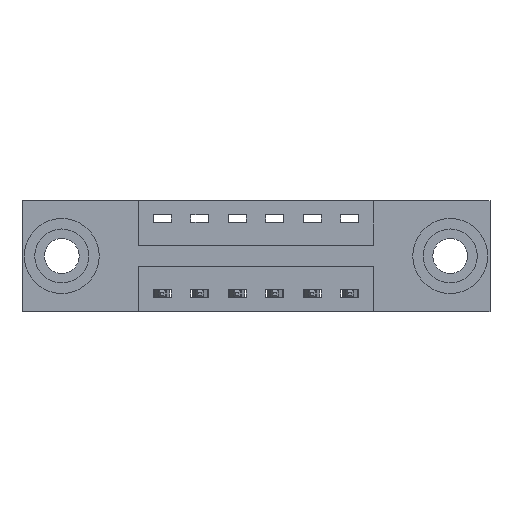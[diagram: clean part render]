
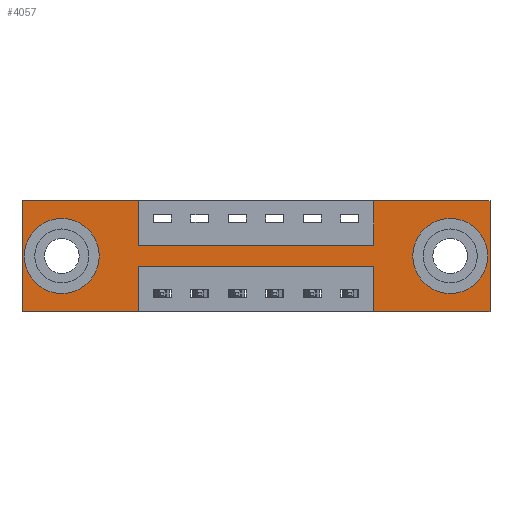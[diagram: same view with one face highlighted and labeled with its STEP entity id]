
A CAD part, front view. The second image highlights one B-rep face of the part: STEP entity #4057.
In plain terms, the highlighted planar face has unit normal (0, -1, 0).
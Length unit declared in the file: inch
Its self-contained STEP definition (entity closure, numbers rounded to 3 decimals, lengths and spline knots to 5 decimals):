
#3 = LINE ( 'NONE', #8240, #7728 ) ;
#8 = EDGE_CURVE ( 'NONE', #4295, #1855, #4288, .T. ) ;
#44 = FACE_OUTER_BOUND ( 'NONE', #9190, .T. ) ;
#78 = CARTESIAN_POINT ( 'NONE',  ( 1.4275, 0., -0.185 ) ) ;
#266 = EDGE_CURVE ( 'NONE', #8594, #5827, #3, .T. ) ;
#280 = LINE ( 'NONE', #2254, #2252 ) ;
#347 = AXIS2_PLACEMENT_3D ( 'NONE', #8436, #8417, #8403 ) ;
#463 = DIRECTION ( 'NONE',  ( 1., 0., 0. ) ) ;
#467 = LINE ( 'NONE', #4411, #4174 ) ;
#488 = LINE ( 'NONE', #4860, #4196 ) ;
#527 = VECTOR ( 'NONE', #7187, 39.37008 ) ;
#554 = CARTESIAN_POINT ( 'NONE',  ( 1.1725, 0., -0.37 ) ) ;
#571 = VERTEX_POINT ( 'NONE', #1957 ) ;
#653 = LINE ( 'NONE', #4208, #8131 ) ;
#664 = VERTEX_POINT ( 'NONE', #9116 ) ;
#706 = EDGE_CURVE ( 'NONE', #1855, #4295, #7501, .T. ) ;
#802 = CARTESIAN_POINT ( 'NONE',  ( 1.1725, 0., 0. ) ) ;
#817 = DIRECTION ( 'NONE',  ( 0., 0., -1. ) ) ;
#831 = ORIENTED_EDGE ( 'NONE', *, *, #8219, .F. ) ;
#1064 = ORIENTED_EDGE ( 'NONE', *, *, #6655, .F. ) ;
#1213 = EDGE_CURVE ( 'NONE', #1971, #5287, #467, .T. ) ;
#1297 = CARTESIAN_POINT ( 'NONE',  ( 0.3875, 0., -0.37 ) ) ;
#1302 = ORIENTED_EDGE ( 'NONE', *, *, #6002, .F. ) ;
#1307 = EDGE_LOOP ( 'NONE', ( #4530, #8278 ) ) ;
#1536 = ORIENTED_EDGE ( 'NONE', *, *, #266, .F. ) ;
#1554 = DIRECTION ( 'NONE',  ( 0., 0., 1. ) ) ;
#1693 = CARTESIAN_POINT ( 'NONE',  ( 1.4275, 0., -0.263 ) ) ;
#1702 = LINE ( 'NONE', #1297, #9037 ) ;
#1736 = AXIS2_PLACEMENT_3D ( 'NONE', #7558, #1827, #6892 ) ;
#1797 = VECTOR ( 'NONE', #4024, 39.37008 ) ;
#1799 = CARTESIAN_POINT ( 'NONE',  ( 0., 0., 0. ) ) ;
#1827 = DIRECTION ( 'NONE',  ( 0., -1., 0. ) ) ;
#1855 = VERTEX_POINT ( 'NONE', #7482 ) ;
#1957 = CARTESIAN_POINT ( 'NONE',  ( 1.1725, 0., -0.15 ) ) ;
#1971 = VERTEX_POINT ( 'NONE', #6198 ) ;
#2047 = LINE ( 'NONE', #802, #2281 ) ;
#2185 = CARTESIAN_POINT ( 'NONE',  ( 0.3875, 0., -0.22 ) ) ;
#2252 = VECTOR ( 'NONE', #2951, 39.37008 ) ;
#2254 = CARTESIAN_POINT ( 'NONE',  ( 0.3875, 0., -0.22 ) ) ;
#2281 = VECTOR ( 'NONE', #1554, 39.37008 ) ;
#2592 = ORIENTED_EDGE ( 'NONE', *, *, #7320, .T. ) ;
#2689 = EDGE_CURVE ( 'NONE', #5827, #7892, #6380, .T. ) ;
#2800 = DIRECTION ( 'NONE',  ( 0., 1., 0. ) ) ;
#2801 = ORIENTED_EDGE ( 'NONE', *, *, #5075, .F. ) ;
#2951 = DIRECTION ( 'NONE',  ( -1., 0., 0. ) ) ;
#3031 = CARTESIAN_POINT ( 'NONE',  ( 0., 0., -0.37 ) ) ;
#3075 = DIRECTION ( 'NONE',  ( 0., 0., -1. ) ) ;
#3173 = VECTOR ( 'NONE', #6745, 39.37008 ) ;
#3273 = ORIENTED_EDGE ( 'NONE', *, *, #3929, .F. ) ;
#3624 = VERTEX_POINT ( 'NONE', #1693 ) ;
#3750 = LINE ( 'NONE', #6861, #1797 ) ;
#3781 = DIRECTION ( 'NONE',  ( -1., 0., 0. ) ) ;
#3860 = AXIS2_PLACEMENT_3D ( 'NONE', #8392, #7022, #7272 ) ;
#3880 = CARTESIAN_POINT ( 'NONE',  ( 0.3875, 0., 0. ) ) ;
#3929 = EDGE_CURVE ( 'NONE', #7003, #8350, #8394, .T. ) ;
#3957 = CARTESIAN_POINT ( 'NONE',  ( 0., 0., -0.37 ) ) ;
#3998 = CARTESIAN_POINT ( 'NONE',  ( 1.56, 0., 0. ) ) ;
#4024 = DIRECTION ( 'NONE',  ( 0., 0., 1. ) ) ;
#4028 = EDGE_CURVE ( 'NONE', #9014, #664, #3750, .T. ) ;
#4051 = LINE ( 'NONE', #3031, #7604 ) ;
#4057 = ADVANCED_FACE ( 'NONE', ( #5455, #7319, #44 ), #5464, .T. ) ;
#4174 = VECTOR ( 'NONE', #4366, 39.37008 ) ;
#4196 = VECTOR ( 'NONE', #463, 39.37008 ) ;
#4208 = CARTESIAN_POINT ( 'NONE',  ( 0., 0., 0. ) ) ;
#4254 = EDGE_CURVE ( 'NONE', #5437, #3624, #7007, .T. ) ;
#4288 = CIRCLE ( 'NONE', #3860, 0.078 ) ;
#4295 = VERTEX_POINT ( 'NONE', #9176 ) ;
#4304 = ORIENTED_EDGE ( 'NONE', *, *, #4254, .T. ) ;
#4366 = DIRECTION ( 'NONE',  ( 1., 0., 0. ) ) ;
#4411 = CARTESIAN_POINT ( 'NONE',  ( 0., 0., 0. ) ) ;
#4530 = ORIENTED_EDGE ( 'NONE', *, *, #706, .T. ) ;
#4860 = CARTESIAN_POINT ( 'NONE',  ( 0.3875, 0., -0.15 ) ) ;
#4975 = ORIENTED_EDGE ( 'NONE', *, *, #5700, .F. ) ;
#4984 = CARTESIAN_POINT ( 'NONE',  ( 1.56, 0., -0.37 ) ) ;
#4988 = AXIS2_PLACEMENT_3D ( 'NONE', #78, #5219, #817 ) ;
#5005 = VERTEX_POINT ( 'NONE', #2185 ) ;
#5075 = EDGE_CURVE ( 'NONE', #664, #5005, #280, .T. ) ;
#5198 = VECTOR ( 'NONE', #3075, 39.37008 ) ;
#5200 = ORIENTED_EDGE ( 'NONE', *, *, #6098, .F. ) ;
#5219 = DIRECTION ( 'NONE',  ( 0., 1., 0. ) ) ;
#5287 = VERTEX_POINT ( 'NONE', #3998 ) ;
#5437 = VERTEX_POINT ( 'NONE', #7661 ) ;
#5455 = FACE_BOUND ( 'NONE', #6465, .T. ) ;
#5464 = PLANE ( 'NONE',  #1736 ) ;
#5700 = EDGE_CURVE ( 'NONE', #5287, #8225, #6663, .T. ) ;
#5827 = VERTEX_POINT ( 'NONE', #3957 ) ;
#6002 = EDGE_CURVE ( 'NONE', #8350, #571, #488, .T. ) ;
#6028 = CARTESIAN_POINT ( 'NONE',  ( 0.3875, 0., -0.37 ) ) ;
#6098 = EDGE_CURVE ( 'NONE', #7892, #7003, #653, .T. ) ;
#6198 = CARTESIAN_POINT ( 'NONE',  ( 1.1725, 0., 0. ) ) ;
#6380 = LINE ( 'NONE', #7225, #527 ) ;
#6465 = EDGE_LOOP ( 'NONE', ( #4304, #2592 ) ) ;
#6655 = EDGE_CURVE ( 'NONE', #8225, #9014, #4051, .T. ) ;
#6663 = LINE ( 'NONE', #7371, #5198 ) ;
#6664 = ORIENTED_EDGE ( 'NONE', *, *, #4028, .F. ) ;
#6745 = DIRECTION ( 'NONE',  ( 0., 0., -1. ) ) ;
#6861 = CARTESIAN_POINT ( 'NONE',  ( 1.1725, 0., -0.37 ) ) ;
#6884 = ORIENTED_EDGE ( 'NONE', *, *, #1213, .F. ) ;
#6892 = DIRECTION ( 'NONE',  ( 0., 0., -1. ) ) ;
#7003 = VERTEX_POINT ( 'NONE', #9045 ) ;
#7007 = CIRCLE ( 'NONE', #7992, 0.078 ) ;
#7022 = DIRECTION ( 'NONE',  ( 0., 1., 0. ) ) ;
#7128 = CARTESIAN_POINT ( 'NONE',  ( 1.4275, 0., -0.185 ) ) ;
#7137 = DIRECTION ( 'NONE',  ( 0., 0., -1. ) ) ;
#7187 = DIRECTION ( 'NONE',  ( 0., 0., 1. ) ) ;
#7190 = CARTESIAN_POINT ( 'NONE',  ( 0.3875, 0., -0.15 ) ) ;
#7225 = CARTESIAN_POINT ( 'NONE',  ( 0., 0., 0. ) ) ;
#7272 = DIRECTION ( 'NONE',  ( 0., 0., 1. ) ) ;
#7319 = FACE_BOUND ( 'NONE', #1307, .T. ) ;
#7320 = EDGE_CURVE ( 'NONE', #3624, #5437, #7478, .T. ) ;
#7371 = CARTESIAN_POINT ( 'NONE',  ( 1.56, 0., 0. ) ) ;
#7478 = CIRCLE ( 'NONE', #4988, 0.078 ) ;
#7482 = CARTESIAN_POINT ( 'NONE',  ( 0.1325, 0., -0.107 ) ) ;
#7501 = CIRCLE ( 'NONE', #347, 0.078 ) ;
#7558 = CARTESIAN_POINT ( 'NONE',  ( 0., 0., -0.37 ) ) ;
#7604 = VECTOR ( 'NONE', #3781, 39.37008 ) ;
#7661 = CARTESIAN_POINT ( 'NONE',  ( 1.4275, 0., -0.107 ) ) ;
#7728 = VECTOR ( 'NONE', #8576, 39.37008 ) ;
#7821 = DIRECTION ( 'NONE',  ( 0., 0., -1. ) ) ;
#7892 = VERTEX_POINT ( 'NONE', #1799 ) ;
#7992 = AXIS2_PLACEMENT_3D ( 'NONE', #7128, #2800, #7821 ) ;
#8131 = VECTOR ( 'NONE', #9080, 39.37008 ) ;
#8219 = EDGE_CURVE ( 'NONE', #5005, #8594, #1702, .T. ) ;
#8225 = VERTEX_POINT ( 'NONE', #4984 ) ;
#8240 = CARTESIAN_POINT ( 'NONE',  ( 0., 0., -0.37 ) ) ;
#8278 = ORIENTED_EDGE ( 'NONE', *, *, #8, .T. ) ;
#8350 = VERTEX_POINT ( 'NONE', #7190 ) ;
#8392 = CARTESIAN_POINT ( 'NONE',  ( 0.1325, 0., -0.185 ) ) ;
#8394 = LINE ( 'NONE', #3880, #3173 ) ;
#8403 = DIRECTION ( 'NONE',  ( 0., 0., 1. ) ) ;
#8417 = DIRECTION ( 'NONE',  ( 0., 1., 0. ) ) ;
#8436 = CARTESIAN_POINT ( 'NONE',  ( 0.1325, 0., -0.185 ) ) ;
#8469 = EDGE_CURVE ( 'NONE', #571, #1971, #2047, .T. ) ;
#8576 = DIRECTION ( 'NONE',  ( -1., 0., 0. ) ) ;
#8594 = VERTEX_POINT ( 'NONE', #6028 ) ;
#8678 = ORIENTED_EDGE ( 'NONE', *, *, #8469, .F. ) ;
#8897 = ORIENTED_EDGE ( 'NONE', *, *, #2689, .F. ) ;
#9014 = VERTEX_POINT ( 'NONE', #554 ) ;
#9037 = VECTOR ( 'NONE', #7137, 39.37008 ) ;
#9045 = CARTESIAN_POINT ( 'NONE',  ( 0.3875, 0., 0. ) ) ;
#9080 = DIRECTION ( 'NONE',  ( 1., 0., 0. ) ) ;
#9116 = CARTESIAN_POINT ( 'NONE',  ( 1.1725, 0., -0.22 ) ) ;
#9176 = CARTESIAN_POINT ( 'NONE',  ( 0.1325, 0., -0.263 ) ) ;
#9190 = EDGE_LOOP ( 'NONE', ( #831, #2801, #6664, #1064, #4975, #6884, #8678, #1302, #3273, #5200, #8897, #1536 ) ) ;
